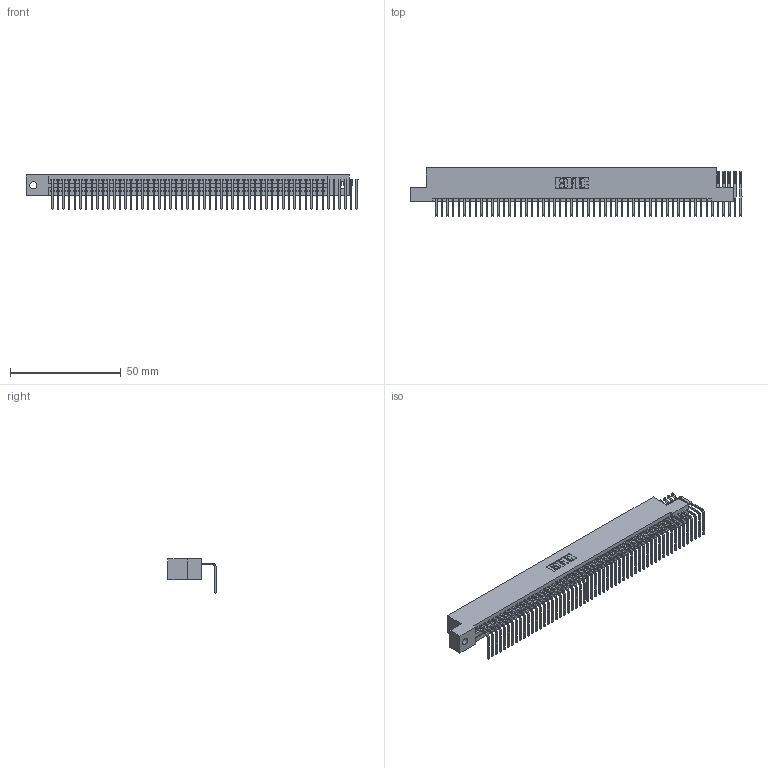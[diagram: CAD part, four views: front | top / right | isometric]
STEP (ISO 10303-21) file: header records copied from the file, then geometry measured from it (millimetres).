
FILE_DESCRIPTION (( 'STEP AP203' ), '1' );
FILE_NAME ('345-055-558-102.STEP', '2019-10-10T19:23:10', ( '' ), ( '' ), 'SwSTEP 2.0', 'SolidWorks 2016', '' );
FILE_SCHEMA (( 'CONFIG_CONTROL_DESIGN' ));
Length unit declared in the file: inch
Products named in the file (3): 345-292-001_558 Tail - 2; 345-055-558-102; 345 Part_Flush Mounting Lugs - 0.128 Dia
Assembly tree (56 placements, depth 2):
  345-055-558-102
    345 Part_Flush Mounting Lugs - 0.128 Dia
    345-292-001_558 Tail - 2  x55
Bounding box: 149.67 x 21.83 x 15.37 mm (x, y, z)
Volume: 14108.4 mm3; surface area: 20014.1 mm2
Topology: 56 solids, 56 shells, 3330 faces, 10027 edges, 6610 vertices
Faces by surface type: plane 2306, cylinder 1024
Entity records: 36215 total; most frequent: CARTESIAN_POINT 6253, ORIENTED_EDGE 6230, DIRECTION 5457, EDGE_CURVE 3115, LINE 2787, VECTOR 2787, VERTEX_POINT 2074, AXIS2_PLACEMENT_3D 1335
